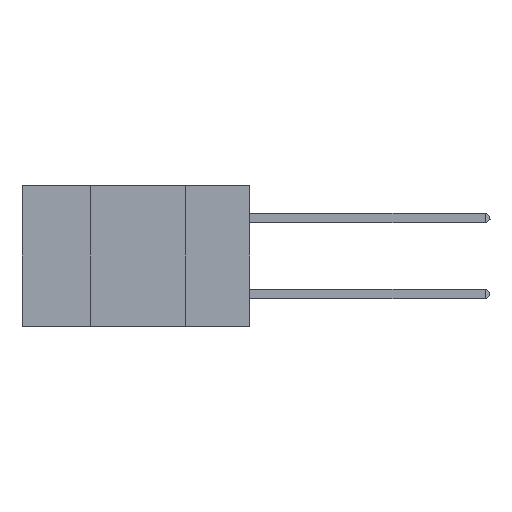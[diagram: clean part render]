
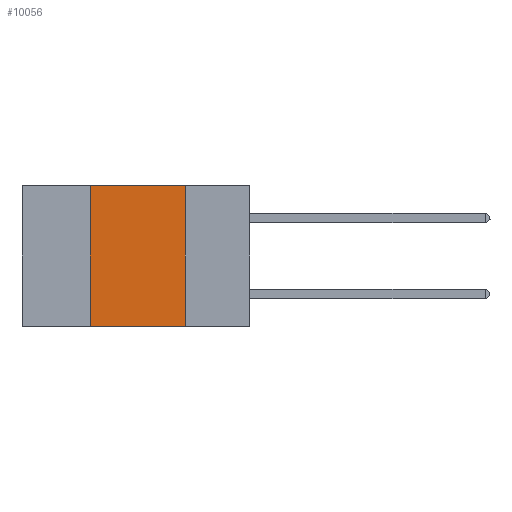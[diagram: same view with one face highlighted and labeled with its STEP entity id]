
A CAD part, left-side view. The second image highlights one B-rep face of the part: STEP entity #10056.
In plain terms, the highlighted planar face has unit normal (-1, 0, 0).
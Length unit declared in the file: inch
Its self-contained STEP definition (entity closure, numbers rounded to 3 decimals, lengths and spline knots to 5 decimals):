
#367 = LINE ( 'NONE', #18398, #14125 ) ;
#1188 = CARTESIAN_POINT ( 'NONE',  ( 0., 0.17, 0. ) ) ;
#1819 = LINE ( 'NONE', #20528, #7588 ) ;
#2059 = DIRECTION ( 'NONE',  ( 0., 0., -1. ) ) ;
#2782 = CARTESIAN_POINT ( 'NONE',  ( 0., 0.42, -0.37 ) ) ;
#2851 = DIRECTION ( 'NONE',  ( 0., -1., 0. ) ) ;
#3080 = LINE ( 'NONE', #6375, #20948 ) ;
#4052 = PLANE ( 'NONE',  #9127 ) ;
#4882 = CARTESIAN_POINT ( 'NONE',  ( 0., 0.17, -0.37 ) ) ;
#5685 = FACE_OUTER_BOUND ( 'NONE', #21411, .T. ) ;
#6375 = CARTESIAN_POINT ( 'NONE',  ( 0., 0.6, -0.37 ) ) ;
#7522 = ORIENTED_EDGE ( 'NONE', *, *, #20126, .T. ) ;
#7588 = VECTOR ( 'NONE', #11622, 39.37008 ) ;
#8267 = ORIENTED_EDGE ( 'NONE', *, *, #8775, .F. ) ;
#8577 = VERTEX_POINT ( 'NONE', #4882 ) ;
#8775 = EDGE_CURVE ( 'NONE', #19555, #20703, #1819, .T. ) ;
#9127 = AXIS2_PLACEMENT_3D ( 'NONE', #14816, #16325, #2059 ) ;
#9372 = DIRECTION ( 'NONE',  ( 0., 0., 1. ) ) ;
#9806 = VERTEX_POINT ( 'NONE', #2782 ) ;
#10056 = ADVANCED_FACE ( 'NONE', ( #5685 ), #4052, .F. ) ;
#10290 = CARTESIAN_POINT ( 'NONE',  ( 0., 0.17, 0. ) ) ;
#11622 = DIRECTION ( 'NONE',  ( 0., -1., 0. ) ) ;
#12298 = VECTOR ( 'NONE', #13916, 39.37008 ) ;
#13916 = DIRECTION ( 'NONE',  ( 0., 0., -1. ) ) ;
#14125 = VECTOR ( 'NONE', #9372, 39.37008 ) ;
#14592 = EDGE_CURVE ( 'NONE', #9806, #19555, #367, .T. ) ;
#14816 = CARTESIAN_POINT ( 'NONE',  ( 0., 0.6, 0. ) ) ;
#15167 = CARTESIAN_POINT ( 'NONE',  ( 0., 0.42, 0. ) ) ;
#16325 = DIRECTION ( 'NONE',  ( 1., 0., 0. ) ) ;
#18398 = CARTESIAN_POINT ( 'NONE',  ( 0., 0.42, 0. ) ) ;
#18842 = EDGE_CURVE ( 'NONE', #20703, #8577, #20953, .T. ) ;
#19555 = VERTEX_POINT ( 'NONE', #15167 ) ;
#20126 = EDGE_CURVE ( 'NONE', #9806, #8577, #3080, .T. ) ;
#20459 = ORIENTED_EDGE ( 'NONE', *, *, #18842, .F. ) ;
#20528 = CARTESIAN_POINT ( 'NONE',  ( 0., 0.6, 0. ) ) ;
#20703 = VERTEX_POINT ( 'NONE', #1188 ) ;
#20948 = VECTOR ( 'NONE', #2851, 39.37008 ) ;
#20953 = LINE ( 'NONE', #10290, #12298 ) ;
#21411 = EDGE_LOOP ( 'NONE', ( #20459, #8267, #22391, #7522 ) ) ;
#22391 = ORIENTED_EDGE ( 'NONE', *, *, #14592, .F. ) ;
